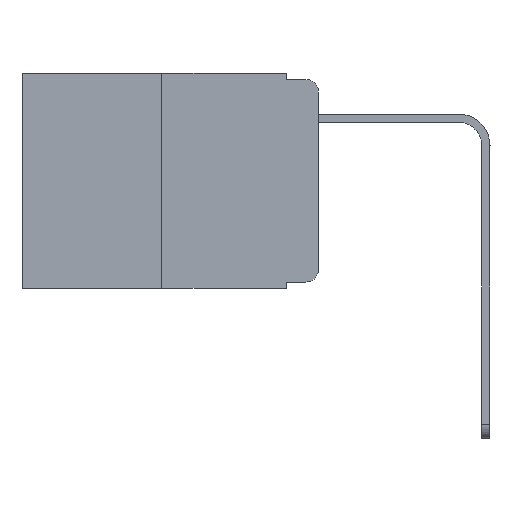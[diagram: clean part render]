
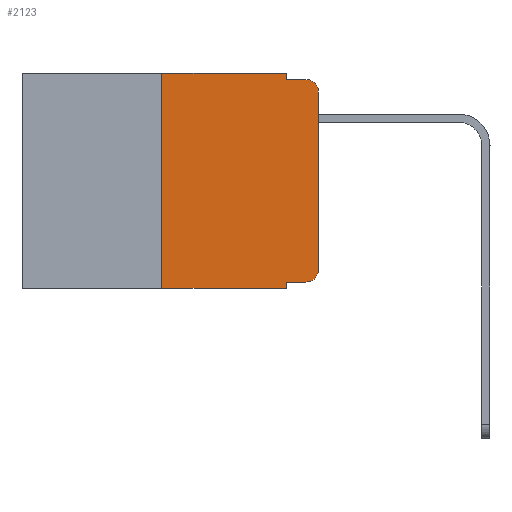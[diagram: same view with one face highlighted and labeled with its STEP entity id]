
A CAD part, left-side view. The second image highlights one B-rep face of the part: STEP entity #2123.
In plain terms, the highlighted planar face has unit normal (-1, 0, 0).
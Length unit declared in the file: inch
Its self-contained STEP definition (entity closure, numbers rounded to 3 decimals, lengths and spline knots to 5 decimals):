
#752 = EDGE_CURVE ( 'NONE', #6715, #3996, #3700, .T. ) ;
#919 = LINE ( 'NONE', #17393, #13582 ) ;
#1158 = CARTESIAN_POINT ( 'NONE',  ( 0., 0.051, -0.333 ) ) ;
#1176 = DIRECTION ( 'NONE',  ( 0., 0., -1. ) ) ;
#1245 = VECTOR ( 'NONE', #11547, 39.37008 ) ;
#1408 = DIRECTION ( 'NONE',  ( -1., 0., 0. ) ) ;
#1438 = EDGE_CURVE ( 'NONE', #9836, #17871, #8082, .T. ) ;
#1757 = DIRECTION ( 'NONE',  ( 0., 0., 1. ) ) ;
#2123 = ADVANCED_FACE ( 'NONE', ( #16859 ), #8621, .F. ) ;
#2666 = CARTESIAN_POINT ( 'NONE',  ( 0., 0.25, -0.343 ) ) ;
#2941 = CARTESIAN_POINT ( 'NONE',  ( 0., 0.051, -0.343 ) ) ;
#3099 = LINE ( 'NONE', #19808, #12354 ) ;
#3230 = LINE ( 'NONE', #13207, #1245 ) ;
#3298 = VERTEX_POINT ( 'NONE', #12094 ) ;
#3700 = LINE ( 'NONE', #17561, #21143 ) ;
#3848 = EDGE_CURVE ( 'NONE', #20186, #5168, #919, .T. ) ;
#3996 = VERTEX_POINT ( 'NONE', #7125 ) ;
#4942 = VECTOR ( 'NONE', #11843, 39.37008 ) ;
#5168 = VERTEX_POINT ( 'NONE', #5862 ) ;
#5862 = CARTESIAN_POINT ( 'NONE',  ( 0., 0.02, -0.01 ) ) ;
#5920 = VECTOR ( 'NONE', #1757, 39.37008 ) ;
#5984 = ORIENTED_EDGE ( 'NONE', *, *, #9652, .F. ) ;
#6589 = CARTESIAN_POINT ( 'NONE',  ( 0., 0., -0.313 ) ) ;
#6715 = VERTEX_POINT ( 'NONE', #2666 ) ;
#6723 = ORIENTED_EDGE ( 'NONE', *, *, #20776, .T. ) ;
#7125 = CARTESIAN_POINT ( 'NONE',  ( 0., 0.25, 0. ) ) ;
#7424 = EDGE_CURVE ( 'NONE', #3298, #9836, #11194, .T. ) ;
#8082 = LINE ( 'NONE', #13477, #5920 ) ;
#8164 = LINE ( 'NONE', #11346, #11809 ) ;
#8517 = EDGE_CURVE ( 'NONE', #6715, #9126, #15584, .T. ) ;
#8621 = PLANE ( 'NONE',  #17462 ) ;
#8749 = ORIENTED_EDGE ( 'NONE', *, *, #1438, .T. ) ;
#8942 = ORIENTED_EDGE ( 'NONE', *, *, #3848, .F. ) ;
#9039 = DIRECTION ( 'NONE',  ( -1., 0., 0. ) ) ;
#9126 = VERTEX_POINT ( 'NONE', #2941 ) ;
#9227 = CARTESIAN_POINT ( 'NONE',  ( 0., 0.051, 0. ) ) ;
#9571 = CARTESIAN_POINT ( 'NONE',  ( 0., 0., -0.03 ) ) ;
#9652 = EDGE_CURVE ( 'NONE', #20330, #20186, #3230, .T. ) ;
#9836 = VERTEX_POINT ( 'NONE', #6589 ) ;
#10700 = DIRECTION ( 'NONE',  ( 0., -1., 0. ) ) ;
#10761 = CARTESIAN_POINT ( 'NONE',  ( 0., 0.02, -0.03 ) ) ;
#10892 = ORIENTED_EDGE ( 'NONE', *, *, #752, .F. ) ;
#11194 = CIRCLE ( 'NONE', #20581, 0.02 ) ;
#11346 = CARTESIAN_POINT ( 'NONE',  ( 0., 0.051, 0. ) ) ;
#11474 = CIRCLE ( 'NONE', #16456, 0.02 ) ;
#11547 = DIRECTION ( 'NONE',  ( 0., 0., -1. ) ) ;
#11809 = VECTOR ( 'NONE', #16594, 39.37008 ) ;
#11843 = DIRECTION ( 'NONE',  ( 0., -1., 0. ) ) ;
#12094 = CARTESIAN_POINT ( 'NONE',  ( 0., 0.02, -0.333 ) ) ;
#12354 = VECTOR ( 'NONE', #10700, 39.37008 ) ;
#13207 = CARTESIAN_POINT ( 'NONE',  ( 0., 0.051, 0. ) ) ;
#13477 = CARTESIAN_POINT ( 'NONE',  ( 0., 0., 0. ) ) ;
#13582 = VECTOR ( 'NONE', #19066, 39.37008 ) ;
#15584 = LINE ( 'NONE', #19784, #4942 ) ;
#15593 = DIRECTION ( 'NONE',  ( 0., 0., -1. ) ) ;
#16006 = EDGE_CURVE ( 'NONE', #17871, #5168, #11474, .T. ) ;
#16456 = AXIS2_PLACEMENT_3D ( 'NONE', #10761, #9039, #21379 ) ;
#16594 = DIRECTION ( 'NONE',  ( 0., 0., -1. ) ) ;
#16595 = EDGE_CURVE ( 'NONE', #3996, #20330, #21880, .T. ) ;
#16859 = FACE_OUTER_BOUND ( 'NONE', #17844, .T. ) ;
#17393 = CARTESIAN_POINT ( 'NONE',  ( 0., 0.051, -0.01 ) ) ;
#17406 = ORIENTED_EDGE ( 'NONE', *, *, #8517, .T. ) ;
#17462 = AXIS2_PLACEMENT_3D ( 'NONE', #22690, #21051, #15593 ) ;
#17561 = CARTESIAN_POINT ( 'NONE',  ( 0., 0.25, 0. ) ) ;
#17844 = EDGE_LOOP ( 'NONE', ( #8749, #18175, #8942, #5984, #19676, #10892, #17406, #21080, #6723, #21949 ) ) ;
#17871 = VERTEX_POINT ( 'NONE', #9571 ) ;
#18175 = ORIENTED_EDGE ( 'NONE', *, *, #16006, .T. ) ;
#19027 = CARTESIAN_POINT ( 'NONE',  ( 0., 0.02, -0.313 ) ) ;
#19066 = DIRECTION ( 'NONE',  ( 0., -1., 0. ) ) ;
#19396 = DIRECTION ( 'NONE',  ( 0., 0., 1. ) ) ;
#19475 = CARTESIAN_POINT ( 'NONE',  ( 0., 0.473, 0. ) ) ;
#19620 = VECTOR ( 'NONE', #21263, 39.37008 ) ;
#19676 = ORIENTED_EDGE ( 'NONE', *, *, #16595, .F. ) ;
#19784 = CARTESIAN_POINT ( 'NONE',  ( 0., 0.473, -0.343 ) ) ;
#19808 = CARTESIAN_POINT ( 'NONE',  ( 0., 0.051, -0.333 ) ) ;
#20186 = VERTEX_POINT ( 'NONE', #21573 ) ;
#20324 = EDGE_CURVE ( 'NONE', #22987, #9126, #8164, .T. ) ;
#20330 = VERTEX_POINT ( 'NONE', #9227 ) ;
#20581 = AXIS2_PLACEMENT_3D ( 'NONE', #19027, #1408, #1176 ) ;
#20776 = EDGE_CURVE ( 'NONE', #22987, #3298, #3099, .T. ) ;
#21051 = DIRECTION ( 'NONE',  ( 1., 0., 0. ) ) ;
#21080 = ORIENTED_EDGE ( 'NONE', *, *, #20324, .F. ) ;
#21143 = VECTOR ( 'NONE', #19396, 39.37008 ) ;
#21263 = DIRECTION ( 'NONE',  ( 0., -1., 0. ) ) ;
#21379 = DIRECTION ( 'NONE',  ( 0., 0., -1. ) ) ;
#21573 = CARTESIAN_POINT ( 'NONE',  ( 0., 0.051, -0.01 ) ) ;
#21880 = LINE ( 'NONE', #19475, #19620 ) ;
#21949 = ORIENTED_EDGE ( 'NONE', *, *, #7424, .T. ) ;
#22690 = CARTESIAN_POINT ( 'NONE',  ( 0., 0.473, 0. ) ) ;
#22987 = VERTEX_POINT ( 'NONE', #1158 ) ;
